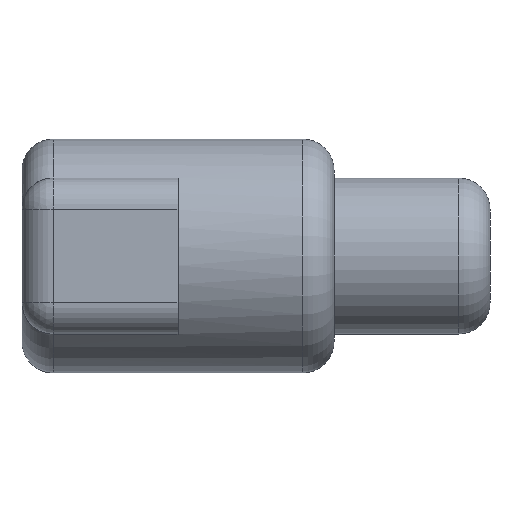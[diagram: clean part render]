
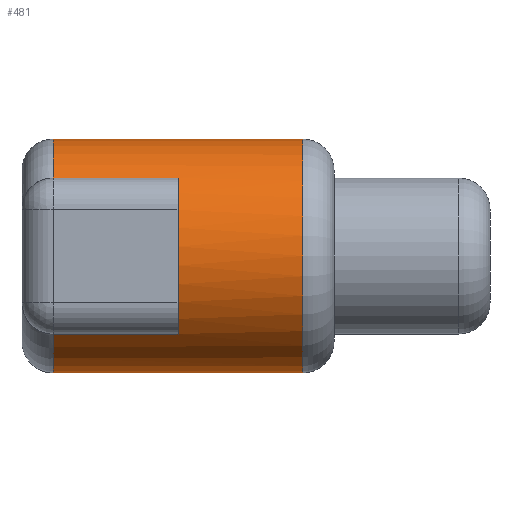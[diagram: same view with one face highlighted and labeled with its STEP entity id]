
A CAD part, left-side view. The second image highlights one B-rep face of the part: STEP entity #481.
In plain terms, the highlighted cylindrical face has radius 7.5 mm (diameter 15 mm), a partial arc.
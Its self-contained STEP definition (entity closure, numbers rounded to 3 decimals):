
#13 = AXIS2_PLACEMENT_3D ( 'NONE', #136, #1064, #395 ) ;
#24 = CARTESIAN_POINT ( 'NONE',  ( 0., 2., -7.5 ) ) ;
#49 = EDGE_CURVE ( 'NONE', #196, #380, #877, .T. ) ;
#57 = VECTOR ( 'NONE', #820, 1000. ) ;
#63 = CARTESIAN_POINT ( 'NONE',  ( -5.59, 18., 5. ) ) ;
#77 = LINE ( 'NONE', #845, #918 ) ;
#90 = DIRECTION ( 'NONE',  ( 0., 0., -1. ) ) ;
#99 = VERTEX_POINT ( 'NONE', #24 ) ;
#116 = DIRECTION ( 'NONE',  ( 0., -1., 0. ) ) ;
#117 = CIRCLE ( 'NONE', #999, 7.5 ) ;
#123 = CIRCLE ( 'NONE', #13, 7.5 ) ;
#131 = EDGE_CURVE ( 'NONE', #99, #414, #123, .T. ) ;
#133 = DIRECTION ( 'NONE',  ( 0., -1., 0. ) ) ;
#136 = CARTESIAN_POINT ( 'NONE',  ( 0., 2., 0. ) ) ;
#149 = CARTESIAN_POINT ( 'NONE',  ( -5.59, 10., 5. ) ) ;
#175 = CARTESIAN_POINT ( 'NONE',  ( 0., 10., 0. ) ) ;
#188 = DIRECTION ( 'NONE',  ( 0., 0., 1. ) ) ;
#192 = CARTESIAN_POINT ( 'NONE',  ( -5.59, 20., 5. ) ) ;
#196 = VERTEX_POINT ( 'NONE', #296 ) ;
#197 = DIRECTION ( 'NONE',  ( 0., -1., 0. ) ) ;
#206 = CARTESIAN_POINT ( 'NONE',  ( 0., 18., 0. ) ) ;
#257 = ORIENTED_EDGE ( 'NONE', *, *, #131, .T. ) ;
#262 = EDGE_CURVE ( 'NONE', #587, #357, #936, .T. ) ;
#269 = CARTESIAN_POINT ( 'NONE',  ( 0., 18., 7.5 ) ) ;
#296 = CARTESIAN_POINT ( 'NONE',  ( -5.59, 10., -5. ) ) ;
#305 = ORIENTED_EDGE ( 'NONE', *, *, #735, .F. ) ;
#307 = VERTEX_POINT ( 'NONE', #149 ) ;
#357 = VERTEX_POINT ( 'NONE', #63 ) ;
#362 = LINE ( 'NONE', #1016, #782 ) ;
#380 = VERTEX_POINT ( 'NONE', #584 ) ;
#395 = DIRECTION ( 'NONE',  ( 0., 0., 1. ) ) ;
#414 = VERTEX_POINT ( 'NONE', #1037 ) ;
#423 = CARTESIAN_POINT ( 'NONE',  ( -5.59, 20., -5. ) ) ;
#466 = ORIENTED_EDGE ( 'NONE', *, *, #984, .T. ) ;
#481 = ADVANCED_FACE ( 'NONE', ( #499 ), #904, .T. ) ;
#499 = FACE_OUTER_BOUND ( 'NONE', #520, .T. ) ;
#520 = EDGE_LOOP ( 'NONE', ( #305, #791, #784, #466, #599, #940, #1042, #257 ) ) ;
#547 = DIRECTION ( 'NONE',  ( 0., 0., 1. ) ) ;
#584 = CARTESIAN_POINT ( 'NONE',  ( -5.59, 18., -5. ) ) ;
#586 = EDGE_CURVE ( 'NONE', #380, #802, #855, .T. ) ;
#587 = VERTEX_POINT ( 'NONE', #269 ) ;
#597 = CARTESIAN_POINT ( 'NONE',  ( 0., 18., -7.5 ) ) ;
#599 = ORIENTED_EDGE ( 'NONE', *, *, #49, .T. ) ;
#607 = AXIS2_PLACEMENT_3D ( 'NONE', #983, #962, #547 ) ;
#638 = AXIS2_PLACEMENT_3D ( 'NONE', #646, #659, #652 ) ;
#646 = CARTESIAN_POINT ( 'NONE',  ( 0., 20., 0. ) ) ;
#652 = DIRECTION ( 'NONE',  ( 0., 0., -1. ) ) ;
#659 = DIRECTION ( 'NONE',  ( 0., -1., 0. ) ) ;
#724 = LINE ( 'NONE', #192, #929 ) ;
#735 = EDGE_CURVE ( 'NONE', #587, #414, #77, .T. ) ;
#782 = VECTOR ( 'NONE', #992, 1000. ) ;
#784 = ORIENTED_EDGE ( 'NONE', *, *, #995, .T. ) ;
#791 = ORIENTED_EDGE ( 'NONE', *, *, #262, .T. ) ;
#802 = VERTEX_POINT ( 'NONE', #597 ) ;
#820 = DIRECTION ( 'NONE',  ( 0., 1., 0. ) ) ;
#845 = CARTESIAN_POINT ( 'NONE',  ( 0., 20., 7.5 ) ) ;
#855 = CIRCLE ( 'NONE', #978, 7.5 ) ;
#877 = LINE ( 'NONE', #423, #57 ) ;
#904 = CYLINDRICAL_SURFACE ( 'NONE', #638, 7.5 ) ;
#905 = DIRECTION ( 'NONE',  ( 0., -1., 0. ) ) ;
#918 = VECTOR ( 'NONE', #905, 1000. ) ;
#929 = VECTOR ( 'NONE', #133, 1000. ) ;
#930 = EDGE_CURVE ( 'NONE', #802, #99, #362, .T. ) ;
#936 = CIRCLE ( 'NONE', #607, 7.5 ) ;
#940 = ORIENTED_EDGE ( 'NONE', *, *, #586, .T. ) ;
#962 = DIRECTION ( 'NONE',  ( 0., -1., 0. ) ) ;
#978 = AXIS2_PLACEMENT_3D ( 'NONE', #206, #197, #188 ) ;
#983 = CARTESIAN_POINT ( 'NONE',  ( 0., 18., 0. ) ) ;
#984 = EDGE_CURVE ( 'NONE', #307, #196, #117, .T. ) ;
#992 = DIRECTION ( 'NONE',  ( 0., -1., 0. ) ) ;
#995 = EDGE_CURVE ( 'NONE', #357, #307, #724, .T. ) ;
#999 = AXIS2_PLACEMENT_3D ( 'NONE', #175, #116, #90 ) ;
#1016 = CARTESIAN_POINT ( 'NONE',  ( 0., 20., -7.5 ) ) ;
#1037 = CARTESIAN_POINT ( 'NONE',  ( 0., 2., 7.5 ) ) ;
#1042 = ORIENTED_EDGE ( 'NONE', *, *, #930, .T. ) ;
#1064 = DIRECTION ( 'NONE',  ( 0., 1., 0. ) ) ;
